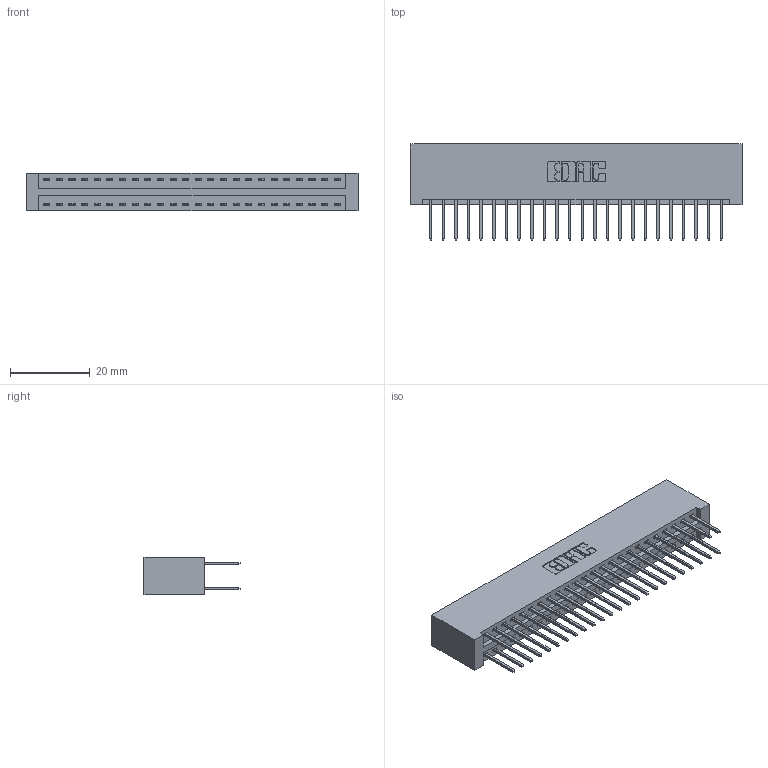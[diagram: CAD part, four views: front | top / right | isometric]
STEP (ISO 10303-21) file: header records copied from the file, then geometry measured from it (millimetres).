
FILE_DESCRIPTION (( 'STEP AP203' ), '1' );
FILE_NAME ('346-048-526-201.STEP', '2018-08-25T09:32:44', ( '' ), ( '' ), 'SwSTEP 2.0', 'SolidWorks 2016', '' );
FILE_SCHEMA (( 'CONFIG_CONTROL_DESIGN' ));
Length unit declared in the file: inch
Products named in the file (3): 346 Part_No Mounting Lugs; 345-292-001_345-293-126; 346-048-526-201
Assembly tree (49 placements, depth 2):
  346-048-526-201
    346 Part_No Mounting Lugs
    345-292-001_345-293-126  x48
Bounding box: 83.44 x 24.13 x 9.4 mm (x, y, z)
Volume: 8648.6 mm3; surface area: 12120.6 mm2
Topology: 49 solids, 49 shells, 2610 faces, 7745 edges, 5098 vertices
Faces by surface type: plane 1752, cylinder 858
Entity records: 17827 total; most frequent: CARTESIAN_POINT 2960, ORIENTED_EDGE 2894, DIRECTION 2655, EDGE_CURVE 1447, VECTOR 1227, LINE 1227, VERTEX_POINT 962, AXIS2_PLACEMENT_3D 714
